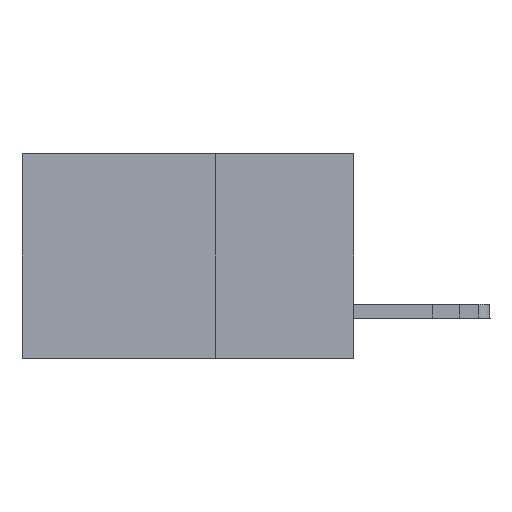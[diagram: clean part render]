
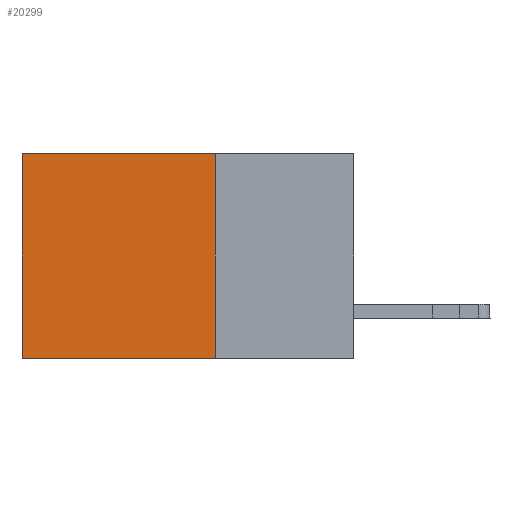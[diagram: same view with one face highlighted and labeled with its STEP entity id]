
A CAD part, left-side view. The second image highlights one B-rep face of the part: STEP entity #20299.
In plain terms, the highlighted planar face has unit normal (-1, 0, 0).
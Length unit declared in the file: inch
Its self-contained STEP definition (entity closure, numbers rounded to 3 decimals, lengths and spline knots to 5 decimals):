
#117 = AXIS2_PLACEMENT_3D ( 'NONE', #12952, #3400, #14466 ) ;
#137 = PLANE ( 'NONE',  #117 ) ;
#1870 = VERTEX_POINT ( 'NONE', #19940 ) ;
#1936 = EDGE_CURVE ( 'NONE', #1870, #3931, #7247, .T. ) ;
#3289 = EDGE_CURVE ( 'NONE', #18252, #13223, #4620, .T. ) ;
#3400 = DIRECTION ( 'NONE',  ( 1., 0., 0. ) ) ;
#3788 = DIRECTION ( 'NONE',  ( 0., 0., -1. ) ) ;
#3931 = VERTEX_POINT ( 'NONE', #13598 ) ;
#4529 = FACE_OUTER_BOUND ( 'NONE', #18776, .T. ) ;
#4620 = LINE ( 'NONE', #18323, #7916 ) ;
#4622 = ORIENTED_EDGE ( 'NONE', *, *, #14687, .T. ) ;
#5324 = ORIENTED_EDGE ( 'NONE', *, *, #18300, .F. ) ;
#6748 = CARTESIAN_POINT ( 'NONE',  ( 0.2875, 0.6, -0.37 ) ) ;
#6876 = DIRECTION ( 'NONE',  ( 0., 1., 0. ) ) ;
#7247 = LINE ( 'NONE', #7637, #11931 ) ;
#7637 = CARTESIAN_POINT ( 'NONE',  ( 0.2875, 0.25, 0. ) ) ;
#7916 = VECTOR ( 'NONE', #16793, 39.37008 ) ;
#10638 = VECTOR ( 'NONE', #6876, 39.37008 ) ;
#11554 = CARTESIAN_POINT ( 'NONE',  ( 0.2875, 0.25, -0.37 ) ) ;
#11931 = VECTOR ( 'NONE', #3788, 39.37008 ) ;
#12952 = CARTESIAN_POINT ( 'NONE',  ( 0.2875, 0.25, 0. ) ) ;
#13087 = CARTESIAN_POINT ( 'NONE',  ( 0.2875, 0.25, 0. ) ) ;
#13223 = VERTEX_POINT ( 'NONE', #6748 ) ;
#13570 = LINE ( 'NONE', #13087, #16650 ) ;
#13598 = CARTESIAN_POINT ( 'NONE',  ( 0.2875, 0.25, -0.37 ) ) ;
#14466 = DIRECTION ( 'NONE',  ( 0., 0., -1. ) ) ;
#14687 = EDGE_CURVE ( 'NONE', #1870, #18252, #13570, .T. ) ;
#16650 = VECTOR ( 'NONE', #17726, 39.37008 ) ;
#16793 = DIRECTION ( 'NONE',  ( 0., 0., -1. ) ) ;
#17006 = ORIENTED_EDGE ( 'NONE', *, *, #3289, .T. ) ;
#17645 = CARTESIAN_POINT ( 'NONE',  ( 0.2875, 0.6, 0. ) ) ;
#17726 = DIRECTION ( 'NONE',  ( 0., 1., 0. ) ) ;
#18127 = ORIENTED_EDGE ( 'NONE', *, *, #1936, .F. ) ;
#18252 = VERTEX_POINT ( 'NONE', #17645 ) ;
#18300 = EDGE_CURVE ( 'NONE', #3931, #13223, #18790, .T. ) ;
#18323 = CARTESIAN_POINT ( 'NONE',  ( 0.2875, 0.6, 0. ) ) ;
#18776 = EDGE_LOOP ( 'NONE', ( #17006, #5324, #18127, #4622 ) ) ;
#18790 = LINE ( 'NONE', #11554, #10638 ) ;
#19940 = CARTESIAN_POINT ( 'NONE',  ( 0.2875, 0.25, 0. ) ) ;
#20299 = ADVANCED_FACE ( 'NONE', ( #4529 ), #137, .F. ) ;
